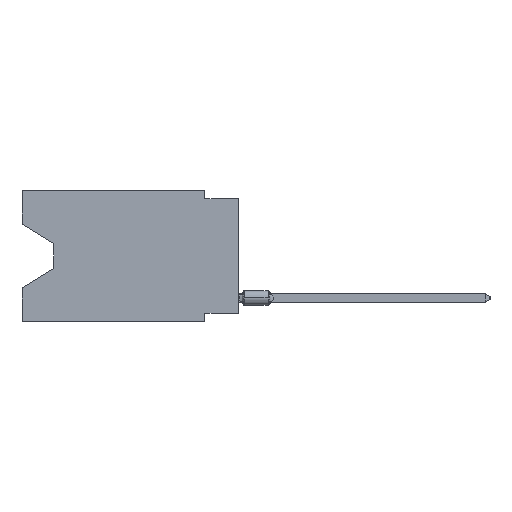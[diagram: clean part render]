
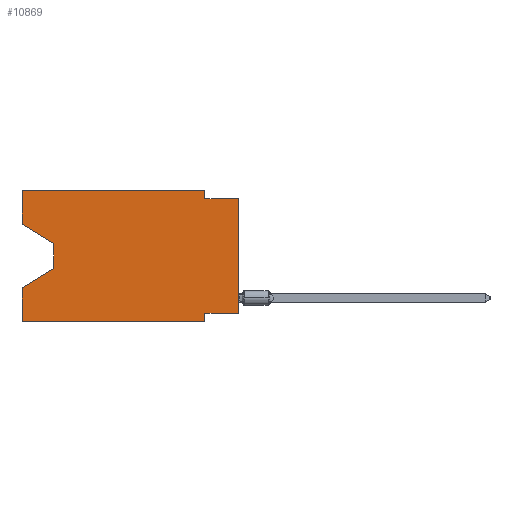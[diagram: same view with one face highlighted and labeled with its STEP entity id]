
A CAD part, left-side view. The second image highlights one B-rep face of the part: STEP entity #10869.
In plain terms, the highlighted planar face has unit normal (-1, 0, 0).
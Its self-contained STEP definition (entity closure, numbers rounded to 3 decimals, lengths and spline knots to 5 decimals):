
#263 = EDGE_CURVE ( 'NONE', #12818, #30228, #21285, .T. ) ;
#700 = VECTOR ( 'NONE', #41107, 39.37008 ) ;
#4044 = EDGE_CURVE ( 'NONE', #13143, #30228, #36894, .T. ) ;
#5521 = LINE ( 'NONE', #44876, #52306 ) ;
#7209 = CARTESIAN_POINT ( 'NONE',  ( 0., 0.1, -0.025 ) ) ;
#7495 = ORIENTED_EDGE ( 'NONE', *, *, #4044, .T. ) ;
#8350 = EDGE_CURVE ( 'NONE', #34707, #22673, #5521, .T. ) ;
#8436 = DIRECTION ( 'NONE',  ( 0., 0., 1. ) ) ;
#9360 = VERTEX_POINT ( 'NONE', #27224 ) ;
#9978 = CARTESIAN_POINT ( 'NONE',  ( 0., 0.645, 0. ) ) ;
#10869 = ADVANCED_FACE ( 'NONE', ( #25376 ), #34894, .F. ) ;
#11599 = DIRECTION ( 'NONE',  ( 0., -1., 0. ) ) ;
#12087 = CARTESIAN_POINT ( 'NONE',  ( 0., 0., -0.365 ) ) ;
#12818 = VERTEX_POINT ( 'NONE', #13760 ) ;
#12895 = VECTOR ( 'NONE', #32295, 39.37008 ) ;
#13115 = VECTOR ( 'NONE', #50980, 39.37008 ) ;
#13143 = VERTEX_POINT ( 'NONE', #39514 ) ;
#13442 = EDGE_CURVE ( 'NONE', #12818, #45333, #27010, .T. ) ;
#13565 = CARTESIAN_POINT ( 'NONE',  ( 0., 0.645, -0.10025 ) ) ;
#13760 = CARTESIAN_POINT ( 'NONE',  ( 0., 0.645, -0.39 ) ) ;
#15720 = CARTESIAN_POINT ( 'NONE',  ( 0., 0.645, 0. ) ) ;
#17187 = VERTEX_POINT ( 'NONE', #18640 ) ;
#17320 = ORIENTED_EDGE ( 'NONE', *, *, #41719, .T. ) ;
#17851 = LINE ( 'NONE', #42773, #12895 ) ;
#18640 = CARTESIAN_POINT ( 'NONE',  ( 0., 0., -0.365 ) ) ;
#19189 = VERTEX_POINT ( 'NONE', #55204 ) ;
#19467 = LINE ( 'NONE', #49645, #40121 ) ;
#21085 = LINE ( 'NONE', #35222, #700 ) ;
#21285 = LINE ( 'NONE', #15720, #59308 ) ;
#21403 = CARTESIAN_POINT ( 'NONE',  ( 0., 0., -0.025 ) ) ;
#22673 = VERTEX_POINT ( 'NONE', #7209 ) ;
#22980 = EDGE_CURVE ( 'NONE', #63419, #13143, #56668, .T. ) ;
#23743 = DIRECTION ( 'NONE',  ( 0., 0., -1. ) ) ;
#24340 = EDGE_LOOP ( 'NONE', ( #48430, #31205, #7495, #55475, #41989, #54183, #39457, #17320, #37690, #40254, #58740, #63590 ) ) ;
#25376 = FACE_OUTER_BOUND ( 'NONE', #24340, .T. ) ;
#26631 = CARTESIAN_POINT ( 'NONE',  ( 0., 0.55, -0.158 ) ) ;
#27010 = LINE ( 'NONE', #47665, #37919 ) ;
#27224 = CARTESIAN_POINT ( 'NONE',  ( 0., 0.1, -0.365 ) ) ;
#27691 = EDGE_CURVE ( 'NONE', #22673, #59227, #17851, .T. ) ;
#29894 = VECTOR ( 'NONE', #57359, 39.37008 ) ;
#30228 = VERTEX_POINT ( 'NONE', #64859 ) ;
#31205 = ORIENTED_EDGE ( 'NONE', *, *, #22980, .T. ) ;
#31725 = EDGE_CURVE ( 'NONE', #17187, #9360, #37363, .T. ) ;
#32213 = CARTESIAN_POINT ( 'NONE',  ( 0., 0.1, 0. ) ) ;
#32295 = DIRECTION ( 'NONE',  ( 0., -1., 0. ) ) ;
#32305 = VECTOR ( 'NONE', #45196, 39.37008 ) ;
#32934 = LINE ( 'NONE', #13565, #36454 ) ;
#33461 = AXIS2_PLACEMENT_3D ( 'NONE', #9978, #45388, #50623 ) ;
#33579 = DIRECTION ( 'NONE',  ( 0., -0.855, -0.519 ) ) ;
#34707 = VERTEX_POINT ( 'NONE', #32213 ) ;
#34894 = PLANE ( 'NONE',  #33461 ) ;
#35222 = CARTESIAN_POINT ( 'NONE',  ( 0., 0., 0. ) ) ;
#35749 = CARTESIAN_POINT ( 'NONE',  ( 0., 0.645, -0.10025 ) ) ;
#36151 = DIRECTION ( 'NONE',  ( 0., 0., -1. ) ) ;
#36454 = VECTOR ( 'NONE', #33579, 39.37008 ) ;
#36894 = LINE ( 'NONE', #46729, #13115 ) ;
#37363 = LINE ( 'NONE', #12087, #29894 ) ;
#37638 = LINE ( 'NONE', #58295, #64282 ) ;
#37690 = ORIENTED_EDGE ( 'NONE', *, *, #27691, .F. ) ;
#37919 = VECTOR ( 'NONE', #11599, 39.37008 ) ;
#39457 = ORIENTED_EDGE ( 'NONE', *, *, #31725, .F. ) ;
#39514 = CARTESIAN_POINT ( 'NONE',  ( 0., 0.55, -0.232 ) ) ;
#40121 = VECTOR ( 'NONE', #23743, 39.37008 ) ;
#40254 = ORIENTED_EDGE ( 'NONE', *, *, #8350, .F. ) ;
#41107 = DIRECTION ( 'NONE',  ( 0., 0., 1. ) ) ;
#41719 = EDGE_CURVE ( 'NONE', #17187, #59227, #21085, .T. ) ;
#41989 = ORIENTED_EDGE ( 'NONE', *, *, #13442, .T. ) ;
#42773 = CARTESIAN_POINT ( 'NONE',  ( 0., 0., -0.025 ) ) ;
#43124 = DIRECTION ( 'NONE',  ( 0., -1., 0. ) ) ;
#43938 = EDGE_CURVE ( 'NONE', #19189, #34707, #63155, .T. ) ;
#44876 = CARTESIAN_POINT ( 'NONE',  ( 0., 0.1, 0. ) ) ;
#45196 = DIRECTION ( 'NONE',  ( 0., 0., -1. ) ) ;
#45333 = VERTEX_POINT ( 'NONE', #46034 ) ;
#45388 = DIRECTION ( 'NONE',  ( 1., 0., 0. ) ) ;
#46034 = CARTESIAN_POINT ( 'NONE',  ( 0., 0.1, -0.39 ) ) ;
#46538 = DIRECTION ( 'NONE',  ( 0., 0., 1. ) ) ;
#46729 = CARTESIAN_POINT ( 'NONE',  ( 0., 0.55, -0.232 ) ) ;
#47665 = CARTESIAN_POINT ( 'NONE',  ( 0., 0.645, -0.39 ) ) ;
#48430 = ORIENTED_EDGE ( 'NONE', *, *, #64446, .T. ) ;
#49645 = CARTESIAN_POINT ( 'NONE',  ( 0., 0.1, -0.39 ) ) ;
#50113 = CARTESIAN_POINT ( 'NONE',  ( 0., 0.55, -0.158 ) ) ;
#50623 = DIRECTION ( 'NONE',  ( 0., 0., -1. ) ) ;
#50980 = DIRECTION ( 'NONE',  ( 0., 0.855, -0.519 ) ) ;
#52306 = VECTOR ( 'NONE', #36151, 39.37008 ) ;
#54183 = ORIENTED_EDGE ( 'NONE', *, *, #60262, .F. ) ;
#55204 = CARTESIAN_POINT ( 'NONE',  ( 0., 0.645, 0. ) ) ;
#55475 = ORIENTED_EDGE ( 'NONE', *, *, #263, .F. ) ;
#56668 = LINE ( 'NONE', #50113, #32305 ) ;
#57359 = DIRECTION ( 'NONE',  ( 0., 1., 0. ) ) ;
#58295 = CARTESIAN_POINT ( 'NONE',  ( 0., 0.645, 0. ) ) ;
#58559 = CARTESIAN_POINT ( 'NONE',  ( 0., 0.645, 0. ) ) ;
#58740 = ORIENTED_EDGE ( 'NONE', *, *, #43938, .F. ) ;
#59227 = VERTEX_POINT ( 'NONE', #21403 ) ;
#59308 = VECTOR ( 'NONE', #46538, 39.37008 ) ;
#59804 = EDGE_CURVE ( 'NONE', #60894, #19189, #37638, .T. ) ;
#60262 = EDGE_CURVE ( 'NONE', #9360, #45333, #19467, .T. ) ;
#60894 = VERTEX_POINT ( 'NONE', #35749 ) ;
#62588 = VECTOR ( 'NONE', #43124, 39.37008 ) ;
#63155 = LINE ( 'NONE', #58559, #62588 ) ;
#63419 = VERTEX_POINT ( 'NONE', #26631 ) ;
#63590 = ORIENTED_EDGE ( 'NONE', *, *, #59804, .F. ) ;
#64282 = VECTOR ( 'NONE', #8436, 39.37008 ) ;
#64446 = EDGE_CURVE ( 'NONE', #60894, #63419, #32934, .T. ) ;
#64859 = CARTESIAN_POINT ( 'NONE',  ( 0., 0.645, -0.28975 ) ) ;
